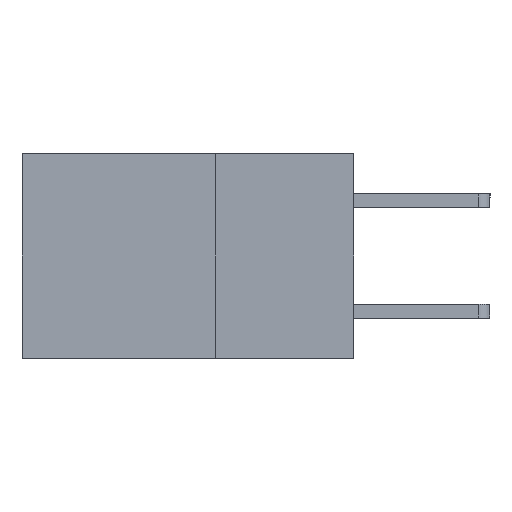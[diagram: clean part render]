
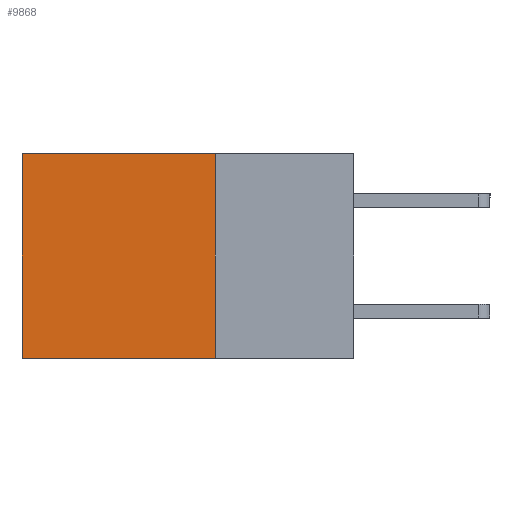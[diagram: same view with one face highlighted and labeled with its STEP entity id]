
A CAD part, left-side view. The second image highlights one B-rep face of the part: STEP entity #9868.
In plain terms, the highlighted planar face has unit normal (-1, 0, 0).
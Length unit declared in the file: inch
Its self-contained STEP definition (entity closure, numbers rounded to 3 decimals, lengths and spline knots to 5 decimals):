
#145 = ORIENTED_EDGE ( 'NONE', *, *, #2775, .F. ) ;
#636 = AXIS2_PLACEMENT_3D ( 'NONE', #4605, #12960, #1517 ) ;
#1517 = DIRECTION ( 'NONE',  ( 0., 0., -1. ) ) ;
#1564 = VERTEX_POINT ( 'NONE', #10023 ) ;
#1837 = CARTESIAN_POINT ( 'NONE',  ( 0.2875, 0.25, -0.37 ) ) ;
#1915 = EDGE_CURVE ( 'NONE', #2791, #2032, #11700, .T. ) ;
#2032 = VERTEX_POINT ( 'NONE', #8888 ) ;
#2507 = DIRECTION ( 'NONE',  ( 0., 0., -1. ) ) ;
#2775 = EDGE_CURVE ( 'NONE', #5520, #1564, #11476, .T. ) ;
#2791 = VERTEX_POINT ( 'NONE', #3895 ) ;
#3549 = LINE ( 'NONE', #11746, #6904 ) ;
#3696 = PLANE ( 'NONE',  #636 ) ;
#3839 = ORIENTED_EDGE ( 'NONE', *, *, #9007, .F. ) ;
#3895 = CARTESIAN_POINT ( 'NONE',  ( 0.2875, 0.25, 0. ) ) ;
#3980 = ORIENTED_EDGE ( 'NONE', *, *, #1915, .T. ) ;
#4537 = FACE_OUTER_BOUND ( 'NONE', #5840, .T. ) ;
#4605 = CARTESIAN_POINT ( 'NONE',  ( 0.2875, 0.25, 0. ) ) ;
#5443 = LINE ( 'NONE', #5577, #8900 ) ;
#5520 = VERTEX_POINT ( 'NONE', #10680 ) ;
#5577 = CARTESIAN_POINT ( 'NONE',  ( 0.2875, 0.6, 0. ) ) ;
#5840 = EDGE_LOOP ( 'NONE', ( #11344, #145, #3839, #3980 ) ) ;
#5854 = VECTOR ( 'NONE', #8412, 39.37008 ) ;
#6904 = VECTOR ( 'NONE', #2507, 39.37008 ) ;
#7662 = DIRECTION ( 'NONE',  ( 0., 0., -1. ) ) ;
#8412 = DIRECTION ( 'NONE',  ( 0., 1., 0. ) ) ;
#8888 = CARTESIAN_POINT ( 'NONE',  ( 0.2875, 0.6, 0. ) ) ;
#8900 = VECTOR ( 'NONE', #7662, 39.37008 ) ;
#9007 = EDGE_CURVE ( 'NONE', #2791, #5520, #3549, .T. ) ;
#9868 = ADVANCED_FACE ( 'NONE', ( #4537 ), #3696, .F. ) ;
#10023 = CARTESIAN_POINT ( 'NONE',  ( 0.2875, 0.6, -0.37 ) ) ;
#10331 = VECTOR ( 'NONE', #10748, 39.37008 ) ;
#10680 = CARTESIAN_POINT ( 'NONE',  ( 0.2875, 0.25, -0.37 ) ) ;
#10748 = DIRECTION ( 'NONE',  ( 0., 1., 0. ) ) ;
#11344 = ORIENTED_EDGE ( 'NONE', *, *, #12293, .T. ) ;
#11476 = LINE ( 'NONE', #1837, #5854 ) ;
#11629 = CARTESIAN_POINT ( 'NONE',  ( 0.2875, 0.25, 0. ) ) ;
#11700 = LINE ( 'NONE', #11629, #10331 ) ;
#11746 = CARTESIAN_POINT ( 'NONE',  ( 0.2875, 0.25, 0. ) ) ;
#12293 = EDGE_CURVE ( 'NONE', #2032, #1564, #5443, .T. ) ;
#12960 = DIRECTION ( 'NONE',  ( 1., 0., 0. ) ) ;
